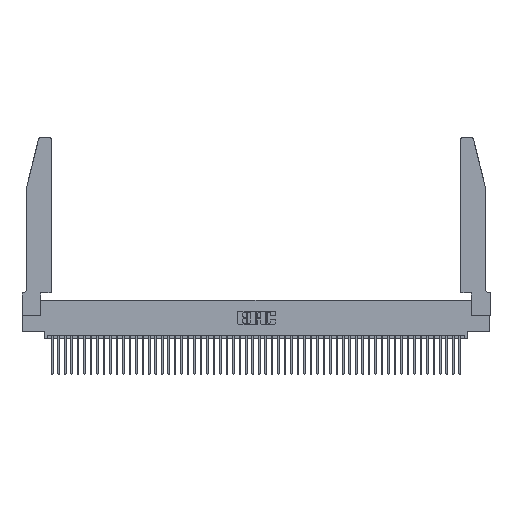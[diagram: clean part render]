
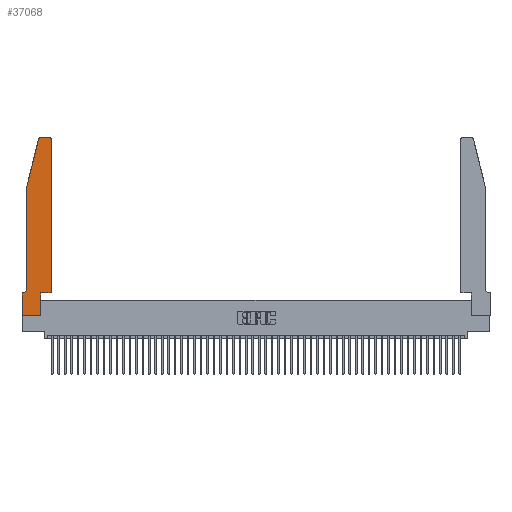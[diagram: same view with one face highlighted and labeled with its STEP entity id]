
A CAD part, top view. The second image highlights one B-rep face of the part: STEP entity #37068.
In plain terms, the highlighted planar face has unit normal (0, 0, 1).
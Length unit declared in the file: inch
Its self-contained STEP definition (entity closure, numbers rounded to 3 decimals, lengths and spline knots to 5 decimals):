
#19 = ORIENTED_EDGE ( 'NONE', *, *, #11093, .T. ) ;
#258 = AXIS2_PLACEMENT_3D ( 'NONE', #1875, #13169, #13338 ) ;
#311 = DIRECTION ( 'NONE',  ( -1., 0., 0. ) ) ;
#655 = LINE ( 'NONE', #1942, #42293 ) ;
#819 = EDGE_CURVE ( 'NONE', #18570, #23755, #24569, .T. ) ;
#1875 = CARTESIAN_POINT ( 'NONE',  ( 0., 0.35, 0.37 ) ) ;
#1942 = CARTESIAN_POINT ( 'NONE',  ( 0.0755, 2., 0.37 ) ) ;
#3084 = VECTOR ( 'NONE', #5434, 39.37008 ) ;
#4619 = EDGE_CURVE ( 'NONE', #25884, #32110, #41738, .T. ) ;
#4843 = VECTOR ( 'NONE', #10678, 39.37008 ) ;
#4847 = VECTOR ( 'NONE', #31502, 39.37008 ) ;
#5434 = DIRECTION ( 'NONE',  ( 0., 1., 0. ) ) ;
#6297 = VERTEX_POINT ( 'NONE', #42324 ) ;
#6379 = CIRCLE ( 'NONE', #7413, 0.03 ) ;
#6773 = CARTESIAN_POINT ( 'NONE',  ( 0., 0., 0.37 ) ) ;
#7152 = EDGE_CURVE ( 'NONE', #6297, #16557, #40151, .T. ) ;
#7186 = CARTESIAN_POINT ( 'NONE',  ( 0.2865, 0.35, 0.37 ) ) ;
#7413 = AXIS2_PLACEMENT_3D ( 'NONE', #27827, #31869, #8032 ) ;
#7580 = ORIENTED_EDGE ( 'NONE', *, *, #43133, .T. ) ;
#8032 = DIRECTION ( 'NONE',  ( 1., 0., 0. ) ) ;
#8069 = CARTESIAN_POINT ( 'NONE',  ( 0.4205, 2.75, 0.37 ) ) ;
#8115 = CARTESIAN_POINT ( 'NONE',  ( 0.2865, 0., 0.37 ) ) ;
#8442 = LINE ( 'NONE', #46686, #23660 ) ;
#9043 = DIRECTION ( 'NONE',  ( -0.239, -0.971, 0. ) ) ;
#10408 = VECTOR ( 'NONE', #311, 39.37008 ) ;
#10678 = DIRECTION ( 'NONE',  ( 1., 0., 0. ) ) ;
#11093 = EDGE_CURVE ( 'NONE', #19563, #28049, #655, .T. ) ;
#12543 = ORIENTED_EDGE ( 'NONE', *, *, #28414, .T. ) ;
#12621 = VERTEX_POINT ( 'NONE', #41198 ) ;
#12884 = CARTESIAN_POINT ( 'NONE',  ( 0.284, 2.72, 0.37 ) ) ;
#13169 = DIRECTION ( 'NONE',  ( 0., 0., 1. ) ) ;
#13194 = ORIENTED_EDGE ( 'NONE', *, *, #4619, .T. ) ;
#13338 = DIRECTION ( 'NONE',  ( 1., 0., 0. ) ) ;
#13883 = DIRECTION ( 'NONE',  ( 0., 1., 0. ) ) ;
#14519 = CARTESIAN_POINT ( 'NONE',  ( 0., 0., 0.37 ) ) ;
#16169 = EDGE_CURVE ( 'NONE', #49616, #18570, #31975, .T. ) ;
#16288 = FACE_OUTER_BOUND ( 'NONE', #51926, .T. ) ;
#16557 = VERTEX_POINT ( 'NONE', #25107 ) ;
#16568 = VECTOR ( 'NONE', #26893, 39.37008 ) ;
#17117 = CARTESIAN_POINT ( 'NONE',  ( 0.25487, 2.72718, 0.37 ) ) ;
#17408 = PLANE ( 'NONE',  #258 ) ;
#18570 = VERTEX_POINT ( 'NONE', #8115 ) ;
#19563 = VERTEX_POINT ( 'NONE', #33959 ) ;
#19696 = ORIENTED_EDGE ( 'NONE', *, *, #32758, .T. ) ;
#20296 = ORIENTED_EDGE ( 'NONE', *, *, #33623, .T. ) ;
#20997 = CARTESIAN_POINT ( 'NONE',  ( 0.2865, 0.35, 0.37 ) ) ;
#21132 = CARTESIAN_POINT ( 'NONE',  ( 0.0055, 0.42, 0.37 ) ) ;
#22294 = DIRECTION ( 'NONE',  ( 0., -1., 0. ) ) ;
#23660 = VECTOR ( 'NONE', #13883, 39.37008 ) ;
#23755 = VERTEX_POINT ( 'NONE', #7186 ) ;
#24569 = LINE ( 'NONE', #20997, #3084 ) ;
#24952 = LINE ( 'NONE', #33102, #10408 ) ;
#25107 = CARTESIAN_POINT ( 'NONE',  ( 0., 0.35, 0.37 ) ) ;
#25199 = DIRECTION ( 'NONE',  ( 0., 0., -1. ) ) ;
#25817 = ORIENTED_EDGE ( 'NONE', *, *, #45598, .T. ) ;
#25884 = VERTEX_POINT ( 'NONE', #38332 ) ;
#26893 = DIRECTION ( 'NONE',  ( 0., -1., 0. ) ) ;
#27328 = CARTESIAN_POINT ( 'NONE',  ( 0., 0., 0.37 ) ) ;
#27827 = CARTESIAN_POINT ( 'NONE',  ( 0.4205, 2.72, 0.37 ) ) ;
#28049 = VERTEX_POINT ( 'NONE', #38740 ) ;
#28414 = EDGE_CURVE ( 'NONE', #12621, #32551, #6379, .T. ) ;
#28822 = DIRECTION ( 'NONE',  ( 1., 0., 0. ) ) ;
#29865 = CARTESIAN_POINT ( 'NONE',  ( 0.0755, 2., 0.37 ) ) ;
#30168 = VECTOR ( 'NONE', #28822, 39.37008 ) ;
#31502 = DIRECTION ( 'NONE',  ( -1., 0., 0. ) ) ;
#31869 = DIRECTION ( 'NONE',  ( 0., 0., 1. ) ) ;
#31975 = LINE ( 'NONE', #14519, #4843 ) ;
#32110 = VERTEX_POINT ( 'NONE', #17117 ) ;
#32356 = ORIENTED_EDGE ( 'NONE', *, *, #16169, .T. ) ;
#32551 = VERTEX_POINT ( 'NONE', #8069 ) ;
#32758 = EDGE_CURVE ( 'NONE', #32551, #25884, #24952, .T. ) ;
#33102 = CARTESIAN_POINT ( 'NONE',  ( 0.2605, 2.75, 0.37 ) ) ;
#33623 = EDGE_CURVE ( 'NONE', #16557, #49616, #39900, .T. ) ;
#33926 = LINE ( 'NONE', #44988, #30168 ) ;
#33959 = CARTESIAN_POINT ( 'NONE',  ( 0.0755, 2., 0.37 ) ) ;
#36859 = DIRECTION ( 'NONE',  ( 0., 0., 1. ) ) ;
#37068 = ADVANCED_FACE ( 'NONE', ( #16288 ), #17408, .T. ) ;
#37838 = VERTEX_POINT ( 'NONE', #47114 ) ;
#38332 = CARTESIAN_POINT ( 'NONE',  ( 0.284, 2.75, 0.37 ) ) ;
#38506 = ORIENTED_EDGE ( 'NONE', *, *, #44461, .T. ) ;
#38740 = CARTESIAN_POINT ( 'NONE',  ( 0.0755, 0.42, 0.37 ) ) ;
#39761 = CARTESIAN_POINT ( 'NONE',  ( 0.0755, 0.35, 0.37 ) ) ;
#39900 = LINE ( 'NONE', #6773, #16568 ) ;
#40151 = LINE ( 'NONE', #39761, #4847 ) ;
#40347 = CIRCLE ( 'NONE', #47661, 0.07 ) ;
#40559 = AXIS2_PLACEMENT_3D ( 'NONE', #12884, #36859, #49013 ) ;
#41198 = CARTESIAN_POINT ( 'NONE',  ( 0.4505, 2.72, 0.37 ) ) ;
#41361 = DIRECTION ( 'NONE',  ( -1., 0., 0. ) ) ;
#41605 = EDGE_CURVE ( 'NONE', #32110, #19563, #44560, .T. ) ;
#41738 = CIRCLE ( 'NONE', #40559, 0.03 ) ;
#42271 = ORIENTED_EDGE ( 'NONE', *, *, #819, .T. ) ;
#42293 = VECTOR ( 'NONE', #22294, 39.37008 ) ;
#42324 = CARTESIAN_POINT ( 'NONE',  ( 0.0055, 0.35, 0.37 ) ) ;
#43133 = EDGE_CURVE ( 'NONE', #37838, #12621, #8442, .T. ) ;
#43476 = ORIENTED_EDGE ( 'NONE', *, *, #7152, .T. ) ;
#44461 = EDGE_CURVE ( 'NONE', #23755, #37838, #33926, .T. ) ;
#44560 = LINE ( 'NONE', #29865, #46502 ) ;
#44988 = CARTESIAN_POINT ( 'NONE',  ( 0.4505, 0.35, 0.37 ) ) ;
#45598 = EDGE_CURVE ( 'NONE', #28049, #6297, #40347, .T. ) ;
#46502 = VECTOR ( 'NONE', #9043, 39.37008 ) ;
#46686 = CARTESIAN_POINT ( 'NONE',  ( 0.4505, 0.35, 0.37 ) ) ;
#47114 = CARTESIAN_POINT ( 'NONE',  ( 0.4505, 0.35, 0.37 ) ) ;
#47661 = AXIS2_PLACEMENT_3D ( 'NONE', #21132, #25199, #41361 ) ;
#49013 = DIRECTION ( 'NONE',  ( 1., 0., 0. ) ) ;
#49196 = ORIENTED_EDGE ( 'NONE', *, *, #41605, .T. ) ;
#49616 = VERTEX_POINT ( 'NONE', #27328 ) ;
#51926 = EDGE_LOOP ( 'NONE', ( #19696, #13194, #49196, #19, #25817, #43476, #20296, #32356, #42271, #38506, #7580, #12543 ) ) ;
